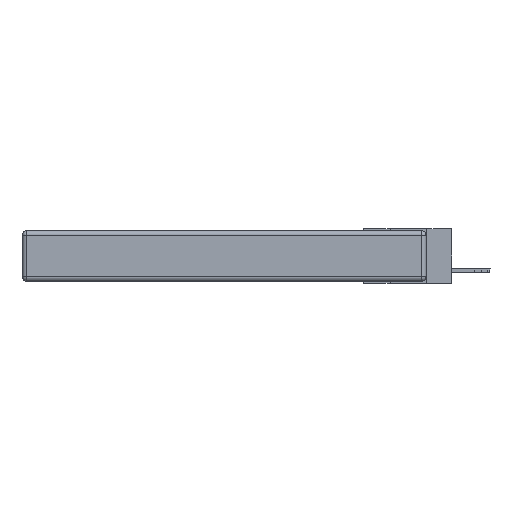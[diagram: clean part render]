
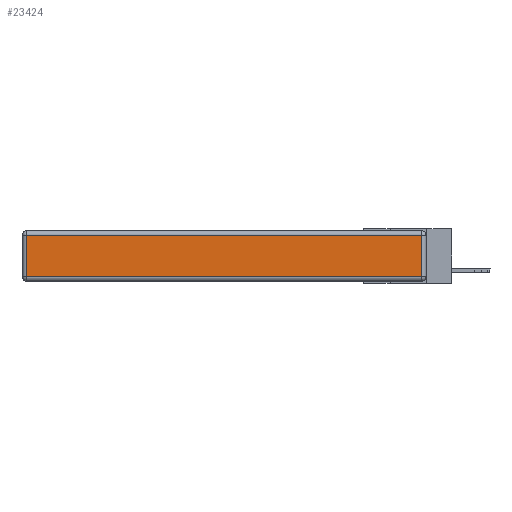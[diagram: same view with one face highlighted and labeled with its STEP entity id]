
A CAD part, left-side view. The second image highlights one B-rep face of the part: STEP entity #23424.
In plain terms, the highlighted planar face has unit normal (-1, 0, 0).
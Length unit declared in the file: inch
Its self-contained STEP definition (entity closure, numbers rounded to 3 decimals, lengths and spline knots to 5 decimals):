
#737 = DIRECTION ( 'NONE',  ( 0., 0., 1. ) ) ;
#1202 = LINE ( 'NONE', #25915, #24504 ) ;
#1543 = LINE ( 'NONE', #4046, #24247 ) ;
#1994 = VERTEX_POINT ( 'NONE', #12556 ) ;
#2470 = EDGE_CURVE ( 'NONE', #1994, #22355, #25515, .T. ) ;
#4046 = CARTESIAN_POINT ( 'NONE',  ( 0., 0.03, -0.343 ) ) ;
#5603 = FACE_OUTER_BOUND ( 'NONE', #12818, .T. ) ;
#5955 = EDGE_CURVE ( 'NONE', #16471, #1994, #1543, .T. ) ;
#7221 = CARTESIAN_POINT ( 'NONE',  ( 0., 0.03, -0.313 ) ) ;
#7700 = EDGE_CURVE ( 'NONE', #15457, #16471, #18139, .T. ) ;
#8633 = CARTESIAN_POINT ( 'NONE',  ( 0., 2.72, -0.03 ) ) ;
#10295 = ORIENTED_EDGE ( 'NONE', *, *, #23039, .T. ) ;
#10676 = CARTESIAN_POINT ( 'NONE',  ( 0., 0., -0.343 ) ) ;
#11071 = CARTESIAN_POINT ( 'NONE',  ( 0., 0., -0.313 ) ) ;
#11514 = CARTESIAN_POINT ( 'NONE',  ( 0., 2.75, -0.03 ) ) ;
#11520 = ORIENTED_EDGE ( 'NONE', *, *, #7700, .T. ) ;
#12556 = CARTESIAN_POINT ( 'NONE',  ( 0., 0.03, -0.03 ) ) ;
#12802 = PLANE ( 'NONE',  #23249 ) ;
#12818 = EDGE_LOOP ( 'NONE', ( #11520, #19711, #14983, #10295 ) ) ;
#14983 = ORIENTED_EDGE ( 'NONE', *, *, #2470, .T. ) ;
#15457 = VERTEX_POINT ( 'NONE', #21985 ) ;
#15459 = VECTOR ( 'NONE', #19590, 39.37008 ) ;
#16471 = VERTEX_POINT ( 'NONE', #7221 ) ;
#18139 = LINE ( 'NONE', #11071, #20030 ) ;
#19590 = DIRECTION ( 'NONE',  ( 0., 1., 0. ) ) ;
#19711 = ORIENTED_EDGE ( 'NONE', *, *, #5955, .T. ) ;
#20030 = VECTOR ( 'NONE', #25058, 39.37008 ) ;
#21985 = CARTESIAN_POINT ( 'NONE',  ( 0., 2.72, -0.313 ) ) ;
#22222 = DIRECTION ( 'NONE',  ( 0., 0., 1. ) ) ;
#22355 = VERTEX_POINT ( 'NONE', #8633 ) ;
#23039 = EDGE_CURVE ( 'NONE', #22355, #15457, #1202, .T. ) ;
#23249 = AXIS2_PLACEMENT_3D ( 'NONE', #10676, #24745, #737 ) ;
#23424 = ADVANCED_FACE ( 'NONE', ( #5603 ), #12802, .T. ) ;
#24247 = VECTOR ( 'NONE', #22222, 39.37008 ) ;
#24504 = VECTOR ( 'NONE', #25484, 39.37008 ) ;
#24745 = DIRECTION ( 'NONE',  ( -1., 0., 0. ) ) ;
#25058 = DIRECTION ( 'NONE',  ( 0., -1., 0. ) ) ;
#25484 = DIRECTION ( 'NONE',  ( 0., 0., -1. ) ) ;
#25515 = LINE ( 'NONE', #11514, #15459 ) ;
#25915 = CARTESIAN_POINT ( 'NONE',  ( 0., 2.72, -0.343 ) ) ;
